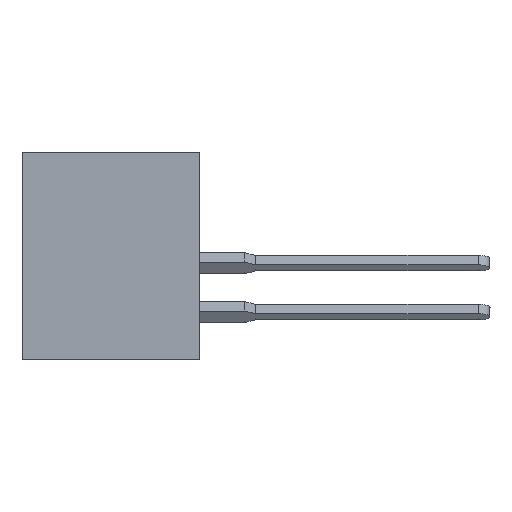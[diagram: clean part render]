
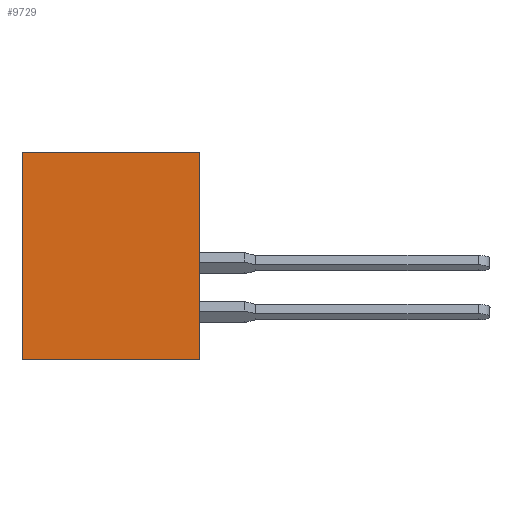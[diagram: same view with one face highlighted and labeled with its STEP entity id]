
A CAD part, left-side view. The second image highlights one B-rep face of the part: STEP entity #9729.
In plain terms, the highlighted planar face has unit normal (-1, 0, 0).
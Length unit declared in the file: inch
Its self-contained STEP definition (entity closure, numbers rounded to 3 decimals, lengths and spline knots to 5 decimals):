
#290 = LINE ( 'NONE', #10053, #22059 ) ;
#690 = ORIENTED_EDGE ( 'NONE', *, *, #18433, .F. ) ;
#1686 = VECTOR ( 'NONE', #14596, 39.37008 ) ;
#2541 = VERTEX_POINT ( 'NONE', #15460 ) ;
#3363 = CARTESIAN_POINT ( 'NONE',  ( 0., 0.453, 0. ) ) ;
#4464 = EDGE_CURVE ( 'NONE', #5108, #2541, #7166, .T. ) ;
#4485 = EDGE_CURVE ( 'NONE', #10242, #2541, #16709, .T. ) ;
#5108 = VERTEX_POINT ( 'NONE', #10635 ) ;
#5420 = DIRECTION ( 'NONE',  ( 0., 0., -1. ) ) ;
#5956 = VECTOR ( 'NONE', #18609, 39.37008 ) ;
#7036 = EDGE_CURVE ( 'NONE', #20307, #10242, #290, .T. ) ;
#7166 = LINE ( 'NONE', #10493, #22829 ) ;
#7722 = ORIENTED_EDGE ( 'NONE', *, *, #7036, .T. ) ;
#8007 = DIRECTION ( 'NONE',  ( 0., -1., 0. ) ) ;
#8422 = AXIS2_PLACEMENT_3D ( 'NONE', #3363, #21686, #5420 ) ;
#9729 = ADVANCED_FACE ( 'NONE', ( #12003 ), #15508, .F. ) ;
#10053 = CARTESIAN_POINT ( 'NONE',  ( 0., 0.453, -0.531 ) ) ;
#10088 = ORIENTED_EDGE ( 'NONE', *, *, #4485, .T. ) ;
#10242 = VERTEX_POINT ( 'NONE', #12237 ) ;
#10299 = ORIENTED_EDGE ( 'NONE', *, *, #4464, .F. ) ;
#10493 = CARTESIAN_POINT ( 'NONE',  ( 0., 0.453, 0. ) ) ;
#10574 = CARTESIAN_POINT ( 'NONE',  ( 0., 0.453, 0. ) ) ;
#10635 = CARTESIAN_POINT ( 'NONE',  ( 0., 0.453, 0. ) ) ;
#10846 = CARTESIAN_POINT ( 'NONE',  ( 0., 0., 0. ) ) ;
#12003 = FACE_OUTER_BOUND ( 'NONE', #18000, .T. ) ;
#12104 = CARTESIAN_POINT ( 'NONE',  ( 0., 0.453, -0.531 ) ) ;
#12237 = CARTESIAN_POINT ( 'NONE',  ( 0., 0., -0.531 ) ) ;
#14596 = DIRECTION ( 'NONE',  ( 0., 0., 1. ) ) ;
#15460 = CARTESIAN_POINT ( 'NONE',  ( 0., 0., 0. ) ) ;
#15508 = PLANE ( 'NONE',  #8422 ) ;
#16709 = LINE ( 'NONE', #10846, #1686 ) ;
#18000 = EDGE_LOOP ( 'NONE', ( #10088, #10299, #690, #7722 ) ) ;
#18433 = EDGE_CURVE ( 'NONE', #20307, #5108, #25780, .T. ) ;
#18609 = DIRECTION ( 'NONE',  ( 0., 0., 1. ) ) ;
#18886 = DIRECTION ( 'NONE',  ( 0., -1., 0. ) ) ;
#20307 = VERTEX_POINT ( 'NONE', #12104 ) ;
#21686 = DIRECTION ( 'NONE',  ( 1., 0., 0. ) ) ;
#22059 = VECTOR ( 'NONE', #8007, 39.37008 ) ;
#22829 = VECTOR ( 'NONE', #18886, 39.37008 ) ;
#25780 = LINE ( 'NONE', #10574, #5956 ) ;
